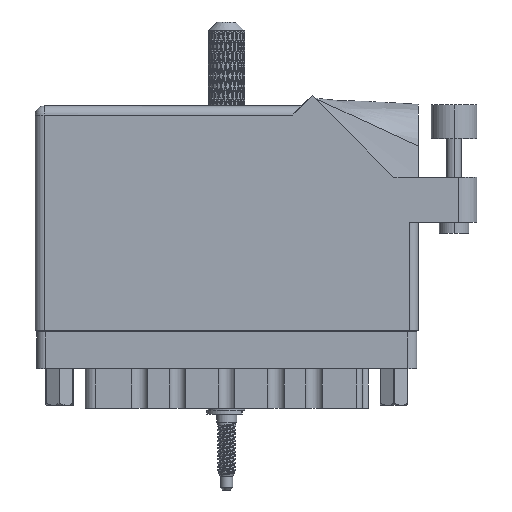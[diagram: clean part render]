
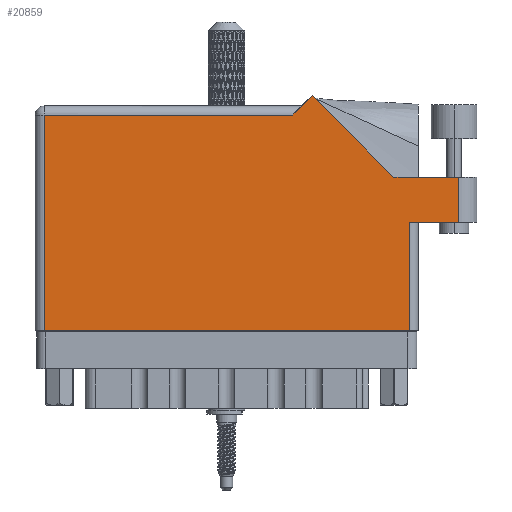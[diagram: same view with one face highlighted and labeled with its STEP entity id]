
A CAD part, front view. The second image highlights one B-rep face of the part: STEP entity #20859.
In plain terms, the highlighted face is planar.
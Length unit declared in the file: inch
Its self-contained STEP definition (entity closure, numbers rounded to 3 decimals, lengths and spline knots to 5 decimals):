
#276 = AXIS2_PLACEMENT_3D ( 'NONE', #121274, #63745, #24612 ) ;
#2604 = VECTOR ( 'NONE', #110435, 39.37008 ) ;
#3842 = VERTEX_POINT ( 'NONE', #78358 ) ;
#4722 = EDGE_CURVE ( 'NONE', #3842, #42564, #104949, .T. ) ;
#5745 = CARTESIAN_POINT ( 'NONE',  ( 1.819, 1.53, 0. ) ) ;
#8392 = ORIENTED_EDGE ( 'NONE', *, *, #76415, .T. ) ;
#10222 = CARTESIAN_POINT ( 'NONE',  ( 2.887, 1.044, 0. ) ) ;
#10991 = VECTOR ( 'NONE', #19839, 39.37008 ) ;
#14187 = LINE ( 'NONE', #58700, #64855 ) ;
#14516 = LINE ( 'NONE', #45419, #95072 ) ;
#14555 = VECTOR ( 'NONE', #64148, 39.37008 ) ;
#17145 = VERTEX_POINT ( 'NONE', #89345 ) ;
#17726 = CARTESIAN_POINT ( 'NONE',  ( 2.44642, 1.044, 0. ) ) ;
#19839 = DIRECTION ( 'NONE',  ( 0., 1., 0. ) ) ;
#20859 = ADVANCED_FACE ( 'NONE', ( #60852 ), #53425, .F. ) ;
#20884 = VERTEX_POINT ( 'NONE', #64156 ) ;
#21286 = CARTESIAN_POINT ( 'NONE',  ( 2.55, 0., 0. ) ) ;
#24612 = DIRECTION ( 'NONE',  ( -1., 0., 0. ) ) ;
#29492 = DIRECTION ( 'NONE',  ( 0., 1., 0. ) ) ;
#32998 = VECTOR ( 'NONE', #71598, 39.37008 ) ;
#34551 = EDGE_CURVE ( 'NONE', #42564, #52663, #102832, .T. ) ;
#39130 = LINE ( 'NONE', #104877, #95760 ) ;
#40155 = EDGE_CURVE ( 'NONE', #119533, #56883, #78649, .T. ) ;
#40499 = LINE ( 'NONE', #76892, #119532 ) ;
#41958 = EDGE_CURVE ( 'NONE', #47867, #3842, #14516, .T. ) ;
#42564 = VERTEX_POINT ( 'NONE', #76323 ) ;
#45419 = CARTESIAN_POINT ( 'NONE',  ( 2.612, 0.737, 0. ) ) ;
#47867 = VERTEX_POINT ( 'NONE', #51146 ) ;
#51146 = CARTESIAN_POINT ( 'NONE',  ( 2.55, 0.737, 0. ) ) ;
#52170 = CARTESIAN_POINT ( 'NONE',  ( 0., 0., 0. ) ) ;
#52663 = VERTEX_POINT ( 'NONE', #17726 ) ;
#53425 = PLANE ( 'NONE',  #276 ) ;
#55580 = ORIENTED_EDGE ( 'NONE', *, *, #89222, .T. ) ;
#56883 = VERTEX_POINT ( 'NONE', #21286 ) ;
#58700 = CARTESIAN_POINT ( 'NONE',  ( 2.55, 0.737, 0. ) ) ;
#60852 = FACE_OUTER_BOUND ( 'NONE', #83086, .T. ) ;
#63745 = DIRECTION ( 'NONE',  ( 0., 0., -1. ) ) ;
#64148 = DIRECTION ( 'NONE',  ( -0.707, 0.707, 0. ) ) ;
#64156 = CARTESIAN_POINT ( 'NONE',  ( 1.757, 1.468, 0. ) ) ;
#64855 = VECTOR ( 'NONE', #29492, 39.37008 ) ;
#66538 = ORIENTED_EDGE ( 'NONE', *, *, #41958, .T. ) ;
#66703 = ORIENTED_EDGE ( 'NONE', *, *, #107487, .T. ) ;
#68654 = ORIENTED_EDGE ( 'NONE', *, *, #111502, .T. ) ;
#71598 = DIRECTION ( 'NONE',  ( -0.707, -0.707, 0. ) ) ;
#72659 = EDGE_CURVE ( 'NONE', #96285, #119533, #40499, .T. ) ;
#76323 = CARTESIAN_POINT ( 'NONE',  ( 2.887, 1.044, 0. ) ) ;
#76415 = EDGE_CURVE ( 'NONE', #52663, #17145, #108474, .T. ) ;
#76892 = CARTESIAN_POINT ( 'NONE',  ( 0.062, 0., 0. ) ) ;
#78358 = CARTESIAN_POINT ( 'NONE',  ( 2.887, 0.737, 0. ) ) ;
#78649 = LINE ( 'NONE', #52170, #2604 ) ;
#83086 = EDGE_LOOP ( 'NONE', ( #66538, #93303, #97435, #8392, #68654, #55580, #99492, #102694, #66703 ) ) ;
#83356 = CARTESIAN_POINT ( 'NONE',  ( 0.062, 0., 0. ) ) ;
#83618 = LINE ( 'NONE', #5745, #32998 ) ;
#84493 = CARTESIAN_POINT ( 'NONE',  ( 2.44642, 1.044, 0. ) ) ;
#89222 = EDGE_CURVE ( 'NONE', #20884, #96285, #39130, .T. ) ;
#89345 = CARTESIAN_POINT ( 'NONE',  ( 1.88971, 1.60071, 0. ) ) ;
#90925 = CARTESIAN_POINT ( 'NONE',  ( 3.012, 1.044, 0. ) ) ;
#93303 = ORIENTED_EDGE ( 'NONE', *, *, #4722, .T. ) ;
#93869 = VECTOR ( 'NONE', #119287, 39.37008 ) ;
#95072 = VECTOR ( 'NONE', #121662, 39.37008 ) ;
#95760 = VECTOR ( 'NONE', #112847, 39.37008 ) ;
#96083 = DIRECTION ( 'NONE',  ( 0., -1., 0. ) ) ;
#96285 = VERTEX_POINT ( 'NONE', #113575 ) ;
#97435 = ORIENTED_EDGE ( 'NONE', *, *, #34551, .T. ) ;
#99492 = ORIENTED_EDGE ( 'NONE', *, *, #72659, .T. ) ;
#102694 = ORIENTED_EDGE ( 'NONE', *, *, #40155, .T. ) ;
#102832 = LINE ( 'NONE', #90925, #93869 ) ;
#104877 = CARTESIAN_POINT ( 'NONE',  ( 0., 1.468, 0. ) ) ;
#104949 = LINE ( 'NONE', #10222, #10991 ) ;
#107487 = EDGE_CURVE ( 'NONE', #56883, #47867, #14187, .T. ) ;
#108474 = LINE ( 'NONE', #84493, #14555 ) ;
#110435 = DIRECTION ( 'NONE',  ( 1., 0., 0. ) ) ;
#111502 = EDGE_CURVE ( 'NONE', #17145, #20884, #83618, .T. ) ;
#112847 = DIRECTION ( 'NONE',  ( -1., 0., 0. ) ) ;
#113575 = CARTESIAN_POINT ( 'NONE',  ( 0.062, 1.468, 0. ) ) ;
#119287 = DIRECTION ( 'NONE',  ( -1., 0., 0. ) ) ;
#119532 = VECTOR ( 'NONE', #96083, 39.37008 ) ;
#119533 = VERTEX_POINT ( 'NONE', #83356 ) ;
#121274 = CARTESIAN_POINT ( 'NONE',  ( 0., 1.53, 0. ) ) ;
#121662 = DIRECTION ( 'NONE',  ( 1., 0., 0. ) ) ;
